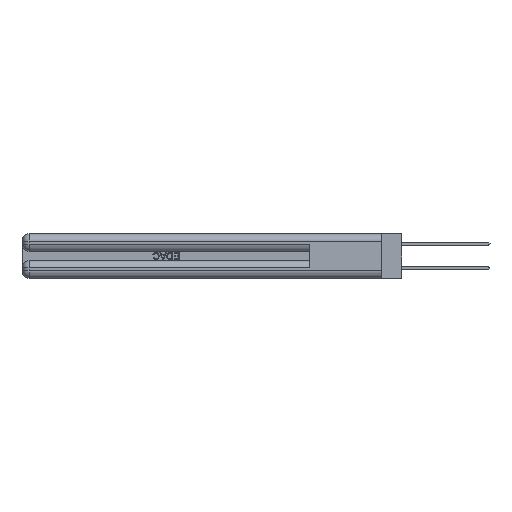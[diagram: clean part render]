
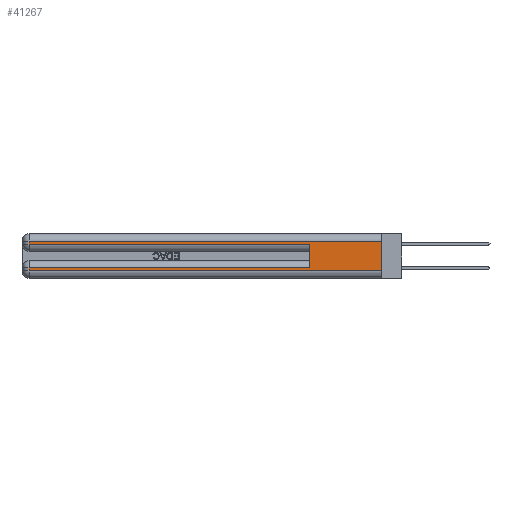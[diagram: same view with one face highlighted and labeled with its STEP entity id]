
A CAD part, left-side view. The second image highlights one B-rep face of the part: STEP entity #41267.
In plain terms, the highlighted planar face has unit normal (-1, 0, 0).
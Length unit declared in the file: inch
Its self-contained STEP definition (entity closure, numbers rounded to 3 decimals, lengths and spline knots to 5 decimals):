
#1498 = ORIENTED_EDGE ( 'NONE', *, *, #48613, .T. ) ;
#2435 = VECTOR ( 'NONE', #28003, 39.37008 ) ;
#2623 = EDGE_CURVE ( 'NONE', #8383, #40717, #32898, .T. ) ;
#2823 = DIRECTION ( 'NONE',  ( 0., 0., -1. ) ) ;
#3291 = VERTEX_POINT ( 'NONE', #34278 ) ;
#3900 = ORIENTED_EDGE ( 'NONE', *, *, #20374, .T. ) ;
#6040 = LINE ( 'NONE', #32712, #33746 ) ;
#8383 = VERTEX_POINT ( 'NONE', #25349 ) ;
#8621 = DIRECTION ( 'NONE',  ( 0., -1., 0. ) ) ;
#11353 = VERTEX_POINT ( 'NONE', #27123 ) ;
#12382 = CARTESIAN_POINT ( 'NONE',  ( 0., 0., 0.31 ) ) ;
#13145 = FACE_OUTER_BOUND ( 'NONE', #24985, .T. ) ;
#13532 = DIRECTION ( 'NONE',  ( 0., 0., -1. ) ) ;
#14805 = DIRECTION ( 'NONE',  ( 0., 0., -1. ) ) ;
#15149 = PLANE ( 'NONE',  #27616 ) ;
#15425 = LINE ( 'NONE', #49920, #27833 ) ;
#16549 = EDGE_CURVE ( 'NONE', #8383, #35224, #38543, .T. ) ;
#18463 = ORIENTED_EDGE ( 'NONE', *, *, #41340, .T. ) ;
#18793 = DIRECTION ( 'NONE',  ( 1., 0., 0. ) ) ;
#19827 = LINE ( 'NONE', #25287, #21077 ) ;
#20148 = DIRECTION ( 'NONE',  ( 0., 1., 0. ) ) ;
#20374 = EDGE_CURVE ( 'NONE', #35224, #33513, #6040, .T. ) ;
#21077 = VECTOR ( 'NONE', #13532, 39.37008 ) ;
#21184 = VECTOR ( 'NONE', #8621, 39.37008 ) ;
#21190 = CARTESIAN_POINT ( 'NONE',  ( 0., 2.94, 0.085 ) ) ;
#23257 = VERTEX_POINT ( 'NONE', #40369 ) ;
#23983 = CARTESIAN_POINT ( 'NONE',  ( 0., 0., 0.285 ) ) ;
#24985 = EDGE_LOOP ( 'NONE', ( #37168, #18463, #29909, #38665, #48828, #27773, #3900, #1498 ) ) ;
#25287 = CARTESIAN_POINT ( 'NONE',  ( 0., 0., 0.37 ) ) ;
#25349 = CARTESIAN_POINT ( 'NONE',  ( 0., 0.6, 0.085 ) ) ;
#27123 = CARTESIAN_POINT ( 'NONE',  ( 0., 0., 0.31 ) ) ;
#27616 = AXIS2_PLACEMENT_3D ( 'NONE', #30526, #18793, #14805 ) ;
#27773 = ORIENTED_EDGE ( 'NONE', *, *, #16549, .T. ) ;
#27833 = VECTOR ( 'NONE', #2823, 39.37008 ) ;
#28003 = DIRECTION ( 'NONE',  ( 0., -1., 0. ) ) ;
#29134 = CARTESIAN_POINT ( 'NONE',  ( 0., 0.6, 0.145 ) ) ;
#29909 = ORIENTED_EDGE ( 'NONE', *, *, #32860, .T. ) ;
#30526 = CARTESIAN_POINT ( 'NONE',  ( 0., 0., 0.37 ) ) ;
#31181 = VERTEX_POINT ( 'NONE', #40456 ) ;
#32712 = CARTESIAN_POINT ( 'NONE',  ( 0., 2.94, 0.37 ) ) ;
#32860 = EDGE_CURVE ( 'NONE', #23257, #3291, #15425, .T. ) ;
#32898 = LINE ( 'NONE', #29134, #38420 ) ;
#33513 = VERTEX_POINT ( 'NONE', #46554 ) ;
#33746 = VECTOR ( 'NONE', #48738, 39.37008 ) ;
#34278 = CARTESIAN_POINT ( 'NONE',  ( 0., 2.94, 0.285 ) ) ;
#35224 = VERTEX_POINT ( 'NONE', #21190 ) ;
#36723 = DIRECTION ( 'NONE',  ( 0., 0., 1. ) ) ;
#37168 = ORIENTED_EDGE ( 'NONE', *, *, #42205, .F. ) ;
#38420 = VECTOR ( 'NONE', #36723, 39.37008 ) ;
#38543 = LINE ( 'NONE', #45360, #42849 ) ;
#38665 = ORIENTED_EDGE ( 'NONE', *, *, #40142, .T. ) ;
#40142 = EDGE_CURVE ( 'NONE', #3291, #40717, #46439, .T. ) ;
#40369 = CARTESIAN_POINT ( 'NONE',  ( 0., 2.94, 0.31 ) ) ;
#40456 = CARTESIAN_POINT ( 'NONE',  ( 0., 0., 0.06 ) ) ;
#40717 = VERTEX_POINT ( 'NONE', #48397 ) ;
#41267 = ADVANCED_FACE ( 'NONE', ( #13145 ), #15149, .F. ) ;
#41340 = EDGE_CURVE ( 'NONE', #11353, #23257, #45840, .T. ) ;
#42205 = EDGE_CURVE ( 'NONE', #11353, #31181, #19827, .T. ) ;
#42849 = VECTOR ( 'NONE', #49344, 39.37008 ) ;
#43158 = LINE ( 'NONE', #47478, #2435 ) ;
#43365 = VECTOR ( 'NONE', #20148, 39.37008 ) ;
#45360 = CARTESIAN_POINT ( 'NONE',  ( 0., 0., 0.085 ) ) ;
#45840 = LINE ( 'NONE', #12382, #43365 ) ;
#46439 = LINE ( 'NONE', #23983, #21184 ) ;
#46554 = CARTESIAN_POINT ( 'NONE',  ( 0., 2.94, 0.06 ) ) ;
#47478 = CARTESIAN_POINT ( 'NONE',  ( 0., 0., 0.06 ) ) ;
#48397 = CARTESIAN_POINT ( 'NONE',  ( 0., 0.6, 0.285 ) ) ;
#48613 = EDGE_CURVE ( 'NONE', #33513, #31181, #43158, .T. ) ;
#48738 = DIRECTION ( 'NONE',  ( 0., 0., -1. ) ) ;
#48828 = ORIENTED_EDGE ( 'NONE', *, *, #2623, .F. ) ;
#49344 = DIRECTION ( 'NONE',  ( 0., 1., 0. ) ) ;
#49920 = CARTESIAN_POINT ( 'NONE',  ( 0., 2.94, 0.37 ) ) ;
